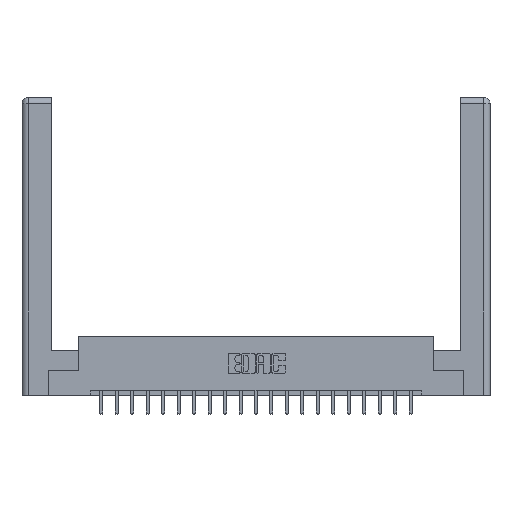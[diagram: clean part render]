
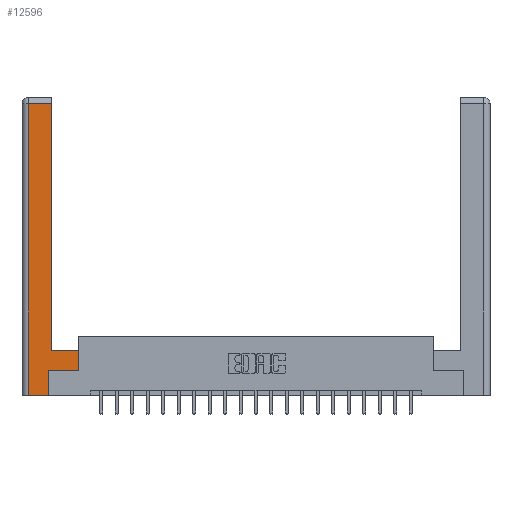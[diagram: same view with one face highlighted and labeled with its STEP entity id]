
A CAD part, top view. The second image highlights one B-rep face of the part: STEP entity #12596.
In plain terms, the highlighted planar face has unit normal (0, 0, 1).
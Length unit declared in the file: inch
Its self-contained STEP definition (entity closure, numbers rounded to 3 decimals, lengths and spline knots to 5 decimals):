
#411 = LINE ( 'NONE', #11763, #3010 ) ;
#499 = CARTESIAN_POINT ( 'NONE',  ( 0.565, 0.245, 0. ) ) ;
#2375 = VECTOR ( 'NONE', #3590, 39.37008 ) ;
#2953 = DIRECTION ( 'NONE',  ( 1., 0., 0. ) ) ;
#3010 = VECTOR ( 'NONE', #13382, 39.37008 ) ;
#3364 = LINE ( 'NONE', #14269, #5480 ) ;
#3590 = DIRECTION ( 'NONE',  ( -1., 0., 0. ) ) ;
#3783 = VERTEX_POINT ( 'NONE', #13345 ) ;
#3886 = DIRECTION ( 'NONE',  ( 0., 1., 0. ) ) ;
#4242 = LINE ( 'NONE', #12324, #12216 ) ;
#4998 = LINE ( 'NONE', #8778, #2375 ) ;
#5069 = CARTESIAN_POINT ( 'NONE',  ( 0.265, 0.245, 0. ) ) ;
#5116 = ORIENTED_EDGE ( 'NONE', *, *, #19398, .T. ) ;
#5151 = DIRECTION ( 'NONE',  ( 0., 0., -1. ) ) ;
#5480 = VECTOR ( 'NONE', #19297, 39.37008 ) ;
#5911 = ORIENTED_EDGE ( 'NONE', *, *, #15011, .T. ) ;
#6820 = CARTESIAN_POINT ( 'NONE',  ( 0.295, 0.45, 0. ) ) ;
#6862 = DIRECTION ( 'NONE',  ( -1., 0., 0. ) ) ;
#7314 = EDGE_CURVE ( 'NONE', #12663, #13875, #17330, .T. ) ;
#8571 = EDGE_CURVE ( 'NONE', #15775, #3783, #15874, .T. ) ;
#8573 = ORIENTED_EDGE ( 'NONE', *, *, #13128, .T. ) ;
#8778 = CARTESIAN_POINT ( 'NONE',  ( 0.0615, 2.94, 0. ) ) ;
#9196 = VECTOR ( 'NONE', #2953, 39.37008 ) ;
#10278 = ORIENTED_EDGE ( 'NONE', *, *, #8571, .T. ) ;
#11379 = CARTESIAN_POINT ( 'NONE',  ( 0.0615, 0., 0. ) ) ;
#11391 = VECTOR ( 'NONE', #13623, 39.37008 ) ;
#11763 = CARTESIAN_POINT ( 'NONE',  ( 0.565, 0.245, 0. ) ) ;
#12020 = LINE ( 'NONE', #11379, #21200 ) ;
#12193 = ORIENTED_EDGE ( 'NONE', *, *, #14040, .T. ) ;
#12216 = VECTOR ( 'NONE', #3886, 39.37008 ) ;
#12220 = VERTEX_POINT ( 'NONE', #18606 ) ;
#12253 = ORIENTED_EDGE ( 'NONE', *, *, #18222, .T. ) ;
#12324 = CARTESIAN_POINT ( 'NONE',  ( 0.295, 3., 0. ) ) ;
#12596 = ADVANCED_FACE ( 'NONE', ( #14267 ), #18619, .F. ) ;
#12605 = CARTESIAN_POINT ( 'NONE',  ( 0.565, 0.45, 0. ) ) ;
#12663 = VERTEX_POINT ( 'NONE', #16857 ) ;
#13128 = EDGE_CURVE ( 'NONE', #12220, #17626, #4998, .T. ) ;
#13152 = LINE ( 'NONE', #5069, #20765 ) ;
#13345 = CARTESIAN_POINT ( 'NONE',  ( 0.295, 0.45, 0. ) ) ;
#13382 = DIRECTION ( 'NONE',  ( 1., 0., 0. ) ) ;
#13584 = CARTESIAN_POINT ( 'NONE',  ( 0., 0., 0. ) ) ;
#13623 = DIRECTION ( 'NONE',  ( -1., 0., 0. ) ) ;
#13790 = CARTESIAN_POINT ( 'NONE',  ( 0.0615, 2.94, 0. ) ) ;
#13875 = VERTEX_POINT ( 'NONE', #14608 ) ;
#14040 = EDGE_CURVE ( 'NONE', #13875, #15059, #13152, .T. ) ;
#14267 = FACE_OUTER_BOUND ( 'NONE', #16889, .T. ) ;
#14269 = CARTESIAN_POINT ( 'NONE',  ( 0.565, 0.45, 0. ) ) ;
#14564 = CARTESIAN_POINT ( 'NONE',  ( 0.265, 0.245, 0. ) ) ;
#14608 = CARTESIAN_POINT ( 'NONE',  ( 0.265, 0., 0. ) ) ;
#15011 = EDGE_CURVE ( 'NONE', #21704, #15775, #3364, .T. ) ;
#15059 = VERTEX_POINT ( 'NONE', #14564 ) ;
#15775 = VERTEX_POINT ( 'NONE', #12605 ) ;
#15874 = LINE ( 'NONE', #6820, #11391 ) ;
#16225 = DIRECTION ( 'NONE',  ( 0., -1., 0. ) ) ;
#16857 = CARTESIAN_POINT ( 'NONE',  ( 0.0615, 0., 0. ) ) ;
#16889 = EDGE_LOOP ( 'NONE', ( #5116, #8573, #12253, #18071, #12193, #18198, #5911, #10278 ) ) ;
#17330 = LINE ( 'NONE', #17892, #9196 ) ;
#17626 = VERTEX_POINT ( 'NONE', #13790 ) ;
#17710 = AXIS2_PLACEMENT_3D ( 'NONE', #13584, #5151, #6862 ) ;
#17892 = CARTESIAN_POINT ( 'NONE',  ( 0.265, 0., 0. ) ) ;
#18071 = ORIENTED_EDGE ( 'NONE', *, *, #7314, .T. ) ;
#18198 = ORIENTED_EDGE ( 'NONE', *, *, #18428, .T. ) ;
#18222 = EDGE_CURVE ( 'NONE', #17626, #12663, #12020, .T. ) ;
#18428 = EDGE_CURVE ( 'NONE', #15059, #21704, #411, .T. ) ;
#18606 = CARTESIAN_POINT ( 'NONE',  ( 0.295, 2.94, 0. ) ) ;
#18619 = PLANE ( 'NONE',  #17710 ) ;
#19297 = DIRECTION ( 'NONE',  ( 0., 1., 0. ) ) ;
#19398 = EDGE_CURVE ( 'NONE', #3783, #12220, #4242, .T. ) ;
#19787 = DIRECTION ( 'NONE',  ( 0., 1., 0. ) ) ;
#20765 = VECTOR ( 'NONE', #19787, 39.37008 ) ;
#21200 = VECTOR ( 'NONE', #16225, 39.37008 ) ;
#21704 = VERTEX_POINT ( 'NONE', #499 ) ;
